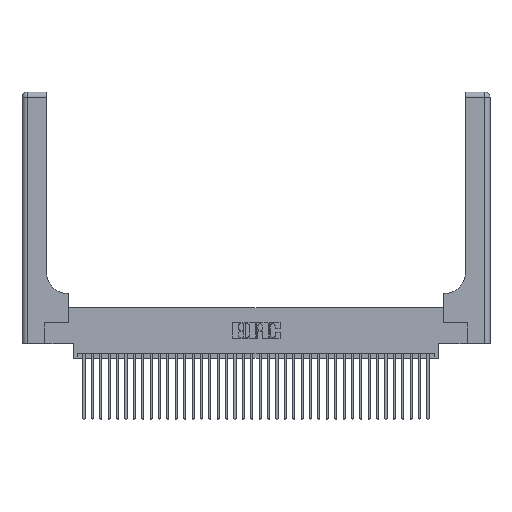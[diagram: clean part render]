
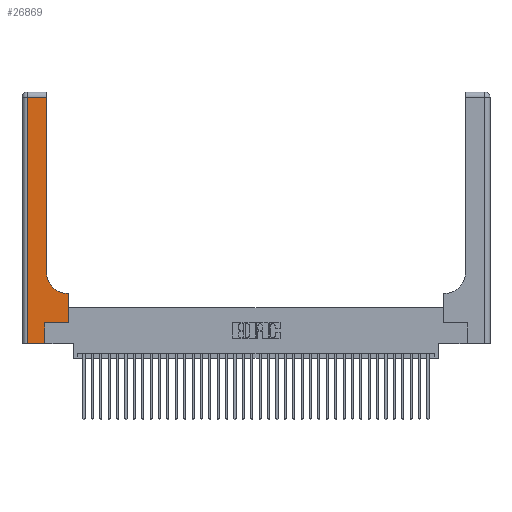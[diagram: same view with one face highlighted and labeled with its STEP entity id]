
A CAD part, top view. The second image highlights one B-rep face of the part: STEP entity #26869.
In plain terms, the highlighted planar face has unit normal (0, 0, 1).
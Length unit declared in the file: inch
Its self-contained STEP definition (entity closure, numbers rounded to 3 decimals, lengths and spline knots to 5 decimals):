
#683 = VECTOR ( 'NONE', #31800, 39.37008 ) ;
#684 = DIRECTION ( 'NONE',  ( -1., 0., 0. ) ) ;
#1036 = AXIS2_PLACEMENT_3D ( 'NONE', #35908, #15120, #684 ) ;
#1642 = VERTEX_POINT ( 'NONE', #28536 ) ;
#1886 = DIRECTION ( 'NONE',  ( 0., 1., 0. ) ) ;
#2249 = ORIENTED_EDGE ( 'NONE', *, *, #33514, .T. ) ;
#2545 = VECTOR ( 'NONE', #33448, 39.37008 ) ;
#2918 = ORIENTED_EDGE ( 'NONE', *, *, #21730, .T. ) ;
#2928 = VECTOR ( 'NONE', #36215, 39.37008 ) ;
#3110 = CARTESIAN_POINT ( 'NONE',  ( 0.269, 0.25, 0.37 ) ) ;
#3497 = CARTESIAN_POINT ( 'NONE',  ( 0.2915, 0.85, 0.37 ) ) ;
#3587 = CARTESIAN_POINT ( 'NONE',  ( 0.269, 0., 0.37 ) ) ;
#4919 = CARTESIAN_POINT ( 'NONE',  ( 0.06, 3., 0.37 ) ) ;
#5536 = VECTOR ( 'NONE', #6558, 39.37008 ) ;
#5835 = CARTESIAN_POINT ( 'NONE',  ( 0.269, 0., 0.37 ) ) ;
#6117 = EDGE_CURVE ( 'NONE', #1642, #33943, #19300, .T. ) ;
#6453 = FACE_OUTER_BOUND ( 'NONE', #22342, .T. ) ;
#6558 = DIRECTION ( 'NONE',  ( 0., 1., 0. ) ) ;
#8214 = VECTOR ( 'NONE', #32947, 39.37008 ) ;
#8278 = VERTEX_POINT ( 'NONE', #10914 ) ;
#8695 = CARTESIAN_POINT ( 'NONE',  ( 0.5415, 0.85, 0.37 ) ) ;
#9271 = PLANE ( 'NONE',  #1036 ) ;
#10914 = CARTESIAN_POINT ( 'NONE',  ( 0.269, 0.25, 0.37 ) ) ;
#12672 = CARTESIAN_POINT ( 'NONE',  ( 0.2915, 0.6, 0.37 ) ) ;
#13242 = CARTESIAN_POINT ( 'NONE',  ( 0.2915, 2.94, 0.37 ) ) ;
#13929 = LINE ( 'NONE', #3587, #5536 ) ;
#14264 = LINE ( 'NONE', #3110, #38289 ) ;
#14357 = CARTESIAN_POINT ( 'NONE',  ( 0.5415, 0.6, 0.37 ) ) ;
#14600 = CARTESIAN_POINT ( 'NONE',  ( 0.5585, 0.25, 0.37 ) ) ;
#15120 = DIRECTION ( 'NONE',  ( 0., 0., -1. ) ) ;
#16075 = CARTESIAN_POINT ( 'NONE',  ( 0.5585, 0.6, 0.37 ) ) ;
#16668 = EDGE_CURVE ( 'NONE', #23225, #1642, #16957, .T. ) ;
#16894 = CIRCLE ( 'NONE', #33052, 0.25 ) ;
#16957 = LINE ( 'NONE', #27031, #2545 ) ;
#17066 = LINE ( 'NONE', #12672, #8214 ) ;
#17898 = ORIENTED_EDGE ( 'NONE', *, *, #30339, .T. ) ;
#19300 = LINE ( 'NONE', #4919, #683 ) ;
#19452 = ORIENTED_EDGE ( 'NONE', *, *, #21784, .T. ) ;
#19599 = VECTOR ( 'NONE', #32152, 39.37008 ) ;
#19689 = CARTESIAN_POINT ( 'NONE',  ( 0.06, 0., 0.37 ) ) ;
#20322 = VERTEX_POINT ( 'NONE', #14600 ) ;
#20530 = LINE ( 'NONE', #32030, #19599 ) ;
#21730 = EDGE_CURVE ( 'NONE', #33825, #38022, #17066, .T. ) ;
#21784 = EDGE_CURVE ( 'NONE', #26118, #8278, #13929, .T. ) ;
#21856 = ORIENTED_EDGE ( 'NONE', *, *, #37917, .T. ) ;
#22342 = EDGE_LOOP ( 'NONE', ( #22764, #23681, #22469, #28908, #19452, #2249, #21856, #2918, #17898 ) ) ;
#22469 = ORIENTED_EDGE ( 'NONE', *, *, #6117, .T. ) ;
#22764 = ORIENTED_EDGE ( 'NONE', *, *, #37944, .T. ) ;
#23225 = VERTEX_POINT ( 'NONE', #13242 ) ;
#23681 = ORIENTED_EDGE ( 'NONE', *, *, #16668, .T. ) ;
#23863 = DIRECTION ( 'NONE',  ( 1., 0., 0. ) ) ;
#26118 = VERTEX_POINT ( 'NONE', #5835 ) ;
#26175 = DIRECTION ( 'NONE',  ( 1., 0., 0. ) ) ;
#26869 = ADVANCED_FACE ( 'NONE', ( #6453 ), #9271, .F. ) ;
#27031 = CARTESIAN_POINT ( 'NONE',  ( 0., 2.94, 0.37 ) ) ;
#28536 = CARTESIAN_POINT ( 'NONE',  ( 0.06, 2.94, 0.37 ) ) ;
#28720 = VERTEX_POINT ( 'NONE', #3497 ) ;
#28908 = ORIENTED_EDGE ( 'NONE', *, *, #30562, .T. ) ;
#30339 = EDGE_CURVE ( 'NONE', #38022, #28720, #16894, .T. ) ;
#30562 = EDGE_CURVE ( 'NONE', #33943, #26118, #33014, .T. ) ;
#31800 = DIRECTION ( 'NONE',  ( 0., -1., 0. ) ) ;
#32030 = CARTESIAN_POINT ( 'NONE',  ( 0.2915, 3., 0.37 ) ) ;
#32052 = LINE ( 'NONE', #34113, #35237 ) ;
#32152 = DIRECTION ( 'NONE',  ( 0., 1., 0. ) ) ;
#32947 = DIRECTION ( 'NONE',  ( -1., 0., 0. ) ) ;
#33014 = LINE ( 'NONE', #36084, #2928 ) ;
#33052 = AXIS2_PLACEMENT_3D ( 'NONE', #8695, #37798, #26175 ) ;
#33448 = DIRECTION ( 'NONE',  ( -1., 0., 0. ) ) ;
#33514 = EDGE_CURVE ( 'NONE', #8278, #20322, #14264, .T. ) ;
#33825 = VERTEX_POINT ( 'NONE', #16075 ) ;
#33943 = VERTEX_POINT ( 'NONE', #19689 ) ;
#34113 = CARTESIAN_POINT ( 'NONE',  ( 0.5585, 0.25, 0.37 ) ) ;
#35237 = VECTOR ( 'NONE', #1886, 39.37008 ) ;
#35908 = CARTESIAN_POINT ( 'NONE',  ( 0., 3., 0.37 ) ) ;
#36084 = CARTESIAN_POINT ( 'NONE',  ( 0., 0., 0.37 ) ) ;
#36215 = DIRECTION ( 'NONE',  ( 1., 0., 0. ) ) ;
#37798 = DIRECTION ( 'NONE',  ( 0., 0., -1. ) ) ;
#37917 = EDGE_CURVE ( 'NONE', #20322, #33825, #32052, .T. ) ;
#37944 = EDGE_CURVE ( 'NONE', #28720, #23225, #20530, .T. ) ;
#38022 = VERTEX_POINT ( 'NONE', #14357 ) ;
#38289 = VECTOR ( 'NONE', #23863, 39.37008 ) ;
